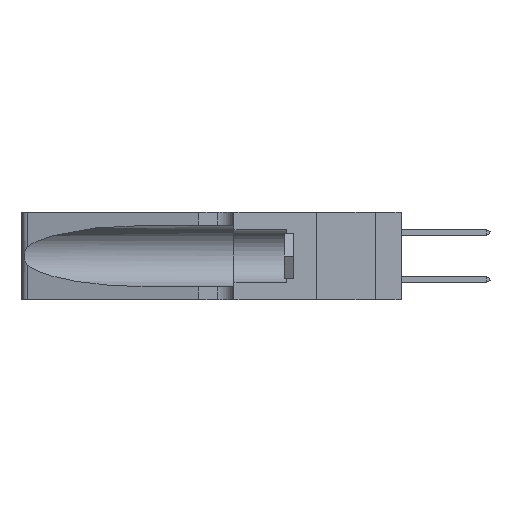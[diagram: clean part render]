
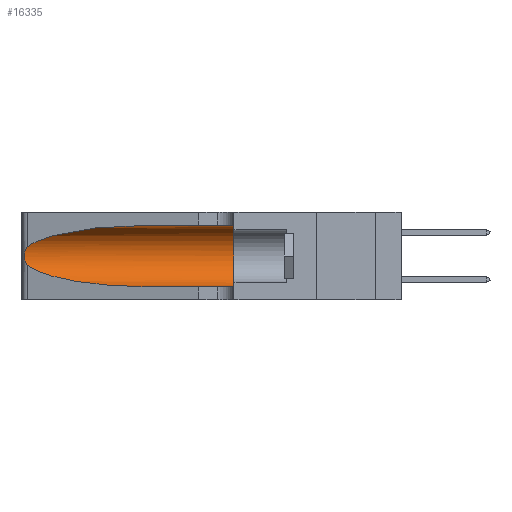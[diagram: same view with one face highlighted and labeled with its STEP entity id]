
A CAD part, left-side view. The second image highlights one B-rep face of the part: STEP entity #16335.
In plain terms, the highlighted cylindrical face has radius 3.308 mm (diameter 6.617 mm), a partial arc.
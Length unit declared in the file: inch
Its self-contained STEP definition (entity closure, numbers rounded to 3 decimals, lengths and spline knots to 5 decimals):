
#1040 = CARTESIAN_POINT ( 'NONE',  ( 0.25487, 1.22718, 0.22369 ) ) ;
#1106 = CARTESIAN_POINT ( 'NONE',  ( 0.1305, 1.61858, 0.185 ) ) ;
#1152 = CARTESIAN_POINT ( 'NONE',  ( 0.25639, 1.23186, 0.15144 ) ) ;
#2407 = DIRECTION ( 'NONE',  ( 0., 1., 0. ) ) ;
#2526 = VERTEX_POINT ( 'NONE', #23660 ) ;
#2638 = CARTESIAN_POINT ( 'NONE',  ( 0.25487, 1.22718, 0.14631 ) ) ;
#3823 = CARTESIAN_POINT ( 'NONE',  ( 0.25487, 1.22718, 0.14631 ) ) ;
#4290 = EDGE_CURVE ( 'NONE', #33434, #33541, #7583, .T. ) ;
#4369 = CARTESIAN_POINT ( 'NONE',  ( 0.25487, 1.22718, 0.14631 ) ) ;
#4692 = EDGE_CURVE ( 'NONE', #33434, #33060, #21909, .T. ) ;
#5224 = FACE_OUTER_BOUND ( 'NONE', #5819, .T. ) ;
#5819 = EDGE_LOOP ( 'NONE', ( #31384, #8194, #31193, #9622, #25091, #25245 ) ) ;
#6351 = CARTESIAN_POINT ( 'NONE',  ( 0.25639, 1.23184, 0.21858 ) ) ;
#7221 = CARTESIAN_POINT ( 'NONE',  ( 0.1305, 1.61858, 0.31525 ) ) ;
#7296 = EDGE_CURVE ( 'NONE', #33541, #17137, #18185, .T. ) ;
#7583 = LINE ( 'NONE', #7221, #27721 ) ;
#7979 = CARTESIAN_POINT ( 'NONE',  ( 0.1305, 0.72297, 0.05475 ) ) ;
#8194 = ORIENTED_EDGE ( 'NONE', *, *, #12750, .T. ) ;
#9022 = CARTESIAN_POINT ( 'NONE',  ( 0.25854, 1.2359, 0.20912 ) ) ;
#9519 = CARTESIAN_POINT ( 'NONE',  ( 0.1305, 0.35, 0.05475 ) ) ;
#9622 = ORIENTED_EDGE ( 'NONE', *, *, #13404, .T. ) ;
#9656 = B_SPLINE_CURVE_WITH_KNOTS ( 'NONE', 3,
 ( #1040, #32484, #6351, #24774, #9022, #27402, #11667, #30009, #14346, #32595, #17018, #1152, #19672, #3823 ),
 .UNSPECIFIED., .F., .F.,
 ( 4, 2, 2, 2, 2, 2, 4 ),
 ( 0., 0.00027, 0.00053, 0.00107, 0.0016, 0.00187, 0.00214 ),
 .UNSPECIFIED. ) ;
#11461 = CARTESIAN_POINT ( 'NONE',  ( 0.18966, 0.96281, 0.31525 ) ) ;
#11667 = CARTESIAN_POINT ( 'NONE',  ( 0.26075, 1.23896, 0.19203 ) ) ;
#11850 = DIRECTION ( 'NONE',  ( 0., -1., 0. ) ) ;
#12750 = EDGE_CURVE ( 'NONE', #33060, #33371, #9656, .T. ) ;
#13092 = EDGE_CURVE ( 'NONE', #33371, #2526, #31479, .T. ) ;
#13404 = EDGE_CURVE ( 'NONE', #2526, #17137, #31084, .T. ) ;
#13753 = CARTESIAN_POINT ( 'NONE',  ( 0.25487, 1.22718, 0.22369 ) ) ;
#14128 = CARTESIAN_POINT ( 'NONE',  ( 0.1305, 0.72297, 0.31525 ) ) ;
#14346 = CARTESIAN_POINT ( 'NONE',  ( 0.26017, 1.23833, 0.17102 ) ) ;
#15083 = DIRECTION ( 'NONE',  ( 0., -1., 0. ) ) ;
#16335 = ADVANCED_FACE ( 'NONE', ( #5224 ), #23766, .F. ) ;
#16800 = CARTESIAN_POINT ( 'NONE',  ( 0.25487, 1.22718, 0.22369 ) ) ;
#17018 = CARTESIAN_POINT ( 'NONE',  ( 0.25789, 1.23486, 0.15765 ) ) ;
#17137 = VERTEX_POINT ( 'NONE', #9519 ) ;
#17198 = VECTOR ( 'NONE', #11850, 39.37008 ) ;
#18185 = CIRCLE ( 'NONE', #32648, 0.13025 ) ;
#18272 = CARTESIAN_POINT ( 'NONE',  ( 0.1305, 0.35, 0.185 ) ) ;
#18501 = CARTESIAN_POINT ( 'NONE',  ( 0.2373, 1.15595, 0.08982 ) ) ;
#19672 = CARTESIAN_POINT ( 'NONE',  ( 0.25555, 1.22993, 0.14849 ) ) ;
#20919 = DIRECTION ( 'NONE',  ( 0., 0., 1. ) ) ;
#21909 =( BOUNDED_CURVE ( )  B_SPLINE_CURVE ( 3, ( #14128, #11461, #32269, #16800 ),
 .UNSPECIFIED., .F., .F. ) 
 B_SPLINE_CURVE_WITH_KNOTS ( ( 4, 4 ),
 ( 1.5708, 2.84003 ),
 .UNSPECIFIED. ) 
 CURVE ( )  GEOMETRIC_REPRESENTATION_ITEM ( )  RATIONAL_B_SPLINE_CURVE ( ( 1., 0.87, 0.87, 1. ) ) 
 REPRESENTATION_ITEM ( '' )  );
#22243 = DIRECTION ( 'NONE',  ( 0., -1., 0. ) ) ;
#23660 = CARTESIAN_POINT ( 'NONE',  ( 0.1305, 0.72297, 0.05475 ) ) ;
#23730 = CARTESIAN_POINT ( 'NONE',  ( 0.18966, 0.96281, 0.05475 ) ) ;
#23766 = CYLINDRICAL_SURFACE ( 'NONE', #24776, 0.13025 ) ;
#24774 = CARTESIAN_POINT ( 'NONE',  ( 0.25787, 1.23484, 0.2124 ) ) ;
#24776 = AXIS2_PLACEMENT_3D ( 'NONE', #1106, #22243, #32546 ) ;
#24961 = CARTESIAN_POINT ( 'NONE',  ( 0.1305, 1.61858, 0.05475 ) ) ;
#25091 = ORIENTED_EDGE ( 'NONE', *, *, #7296, .F. ) ;
#25245 = ORIENTED_EDGE ( 'NONE', *, *, #4290, .F. ) ;
#27402 = CARTESIAN_POINT ( 'NONE',  ( 0.26018, 1.23835, 0.19895 ) ) ;
#27721 = VECTOR ( 'NONE', #15083, 39.37008 ) ;
#28171 = CARTESIAN_POINT ( 'NONE',  ( 0.1305, 0.72297, 0.31525 ) ) ;
#30009 = CARTESIAN_POINT ( 'NONE',  ( 0.26075, 1.23896, 0.178 ) ) ;
#31084 = LINE ( 'NONE', #24961, #17198 ) ;
#31193 = ORIENTED_EDGE ( 'NONE', *, *, #13092, .T. ) ;
#31384 = ORIENTED_EDGE ( 'NONE', *, *, #4692, .T. ) ;
#31479 =( BOUNDED_CURVE ( )  B_SPLINE_CURVE ( 3, ( #2638, #18501, #23730, #7979 ),
 .UNSPECIFIED., .F., .F. ) 
 B_SPLINE_CURVE_WITH_KNOTS ( ( 4, 4 ),
 ( 3.44316, 4.71239 ),
 .UNSPECIFIED. ) 
 CURVE ( )  GEOMETRIC_REPRESENTATION_ITEM ( )  RATIONAL_B_SPLINE_CURVE ( ( 1., 0.87, 0.87, 1. ) ) 
 REPRESENTATION_ITEM ( '' )  );
#32269 = CARTESIAN_POINT ( 'NONE',  ( 0.2373, 1.15595, 0.28018 ) ) ;
#32484 = CARTESIAN_POINT ( 'NONE',  ( 0.25555, 1.22994, 0.2215 ) ) ;
#32546 = DIRECTION ( 'NONE',  ( 0., 0., -1. ) ) ;
#32595 = CARTESIAN_POINT ( 'NONE',  ( 0.25856, 1.23593, 0.16098 ) ) ;
#32648 = AXIS2_PLACEMENT_3D ( 'NONE', #18272, #2407, #20919 ) ;
#33060 = VERTEX_POINT ( 'NONE', #13753 ) ;
#33371 = VERTEX_POINT ( 'NONE', #4369 ) ;
#33434 = VERTEX_POINT ( 'NONE', #28171 ) ;
#33541 = VERTEX_POINT ( 'NONE', #33801 ) ;
#33801 = CARTESIAN_POINT ( 'NONE',  ( 0.1305, 0.35, 0.31525 ) ) ;
